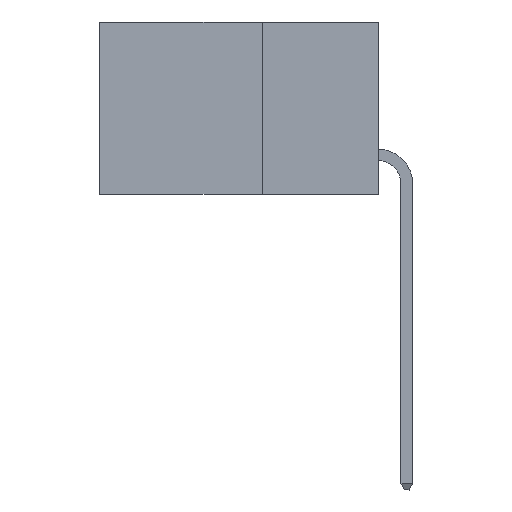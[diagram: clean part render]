
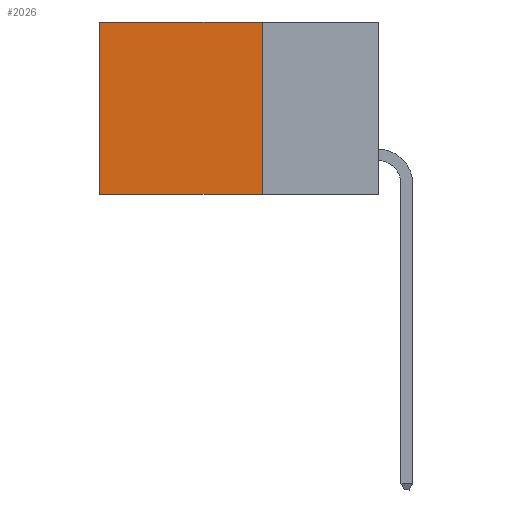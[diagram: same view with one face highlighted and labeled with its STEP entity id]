
A CAD part, left-side view. The second image highlights one B-rep face of the part: STEP entity #2026.
In plain terms, the highlighted planar face has unit normal (-1, 0, 0).
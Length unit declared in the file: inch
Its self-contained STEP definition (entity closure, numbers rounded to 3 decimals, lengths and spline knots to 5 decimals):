
#196 = LINE ( 'NONE', #1033, #2914 ) ;
#475 = CARTESIAN_POINT ( 'NONE',  ( 0.2615, 0.6, -0.37 ) ) ;
#542 = LINE ( 'NONE', #2207, #10078 ) ;
#700 = ORIENTED_EDGE ( 'NONE', *, *, #1999, .F. ) ;
#1033 = CARTESIAN_POINT ( 'NONE',  ( 0.2615, 0.25, -0.37 ) ) ;
#1135 = DIRECTION ( 'NONE',  ( 0., 0., -1. ) ) ;
#1347 = VERTEX_POINT ( 'NONE', #3693 ) ;
#1630 = CARTESIAN_POINT ( 'NONE',  ( 0.2615, 0.25, 0. ) ) ;
#1702 = DIRECTION ( 'NONE',  ( 0., 1., 0. ) ) ;
#1719 = VERTEX_POINT ( 'NONE', #475 ) ;
#1999 = EDGE_CURVE ( 'NONE', #7615, #5984, #196, .T. ) ;
#2026 = ADVANCED_FACE ( 'NONE', ( #4126 ), #8916, .F. ) ;
#2068 = ORIENTED_EDGE ( 'NONE', *, *, #3204, .T. ) ;
#2134 = CARTESIAN_POINT ( 'NONE',  ( 0.2615, 0.25, -0.37 ) ) ;
#2207 = CARTESIAN_POINT ( 'NONE',  ( 0.2615, 0.6, -0.37 ) ) ;
#2288 = EDGE_CURVE ( 'NONE', #5984, #1719, #3723, .T. ) ;
#2914 = VECTOR ( 'NONE', #6529, 39.37008 ) ;
#3204 = EDGE_CURVE ( 'NONE', #7615, #1347, #8104, .T. ) ;
#3693 = CARTESIAN_POINT ( 'NONE',  ( 0.2615, 0.6, 0. ) ) ;
#3723 = LINE ( 'NONE', #6917, #4086 ) ;
#3747 = DIRECTION ( 'NONE',  ( 0., 0., -1. ) ) ;
#3808 = EDGE_CURVE ( 'NONE', #1347, #1719, #542, .T. ) ;
#4086 = VECTOR ( 'NONE', #10101, 39.37008 ) ;
#4126 = FACE_OUTER_BOUND ( 'NONE', #5555, .T. ) ;
#5555 = EDGE_LOOP ( 'NONE', ( #7779, #7881, #700, #2068 ) ) ;
#5773 = CARTESIAN_POINT ( 'NONE',  ( 0.2615, 0.25, 0. ) ) ;
#5984 = VERTEX_POINT ( 'NONE', #2134 ) ;
#6262 = AXIS2_PLACEMENT_3D ( 'NONE', #6587, #7324, #1135 ) ;
#6529 = DIRECTION ( 'NONE',  ( 0., 0., -1. ) ) ;
#6587 = CARTESIAN_POINT ( 'NONE',  ( 0.2615, 0.25, -0.37 ) ) ;
#6917 = CARTESIAN_POINT ( 'NONE',  ( 0.2615, 0.25, -0.37 ) ) ;
#7324 = DIRECTION ( 'NONE',  ( 1., 0., 0. ) ) ;
#7615 = VERTEX_POINT ( 'NONE', #1630 ) ;
#7716 = VECTOR ( 'NONE', #1702, 39.37008 ) ;
#7779 = ORIENTED_EDGE ( 'NONE', *, *, #3808, .T. ) ;
#7881 = ORIENTED_EDGE ( 'NONE', *, *, #2288, .F. ) ;
#8104 = LINE ( 'NONE', #5773, #7716 ) ;
#8916 = PLANE ( 'NONE',  #6262 ) ;
#10078 = VECTOR ( 'NONE', #3747, 39.37008 ) ;
#10101 = DIRECTION ( 'NONE',  ( 0., 1., 0. ) ) ;
